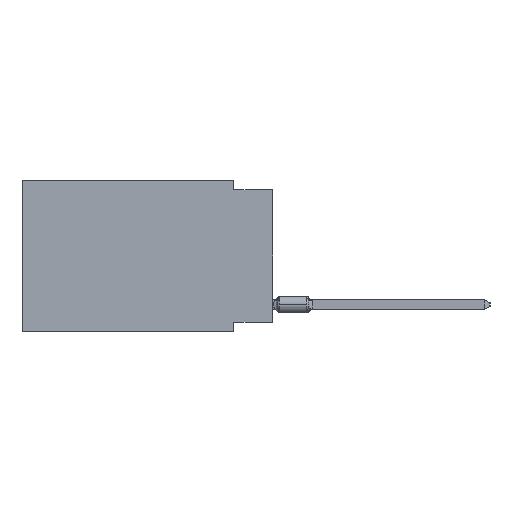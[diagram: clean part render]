
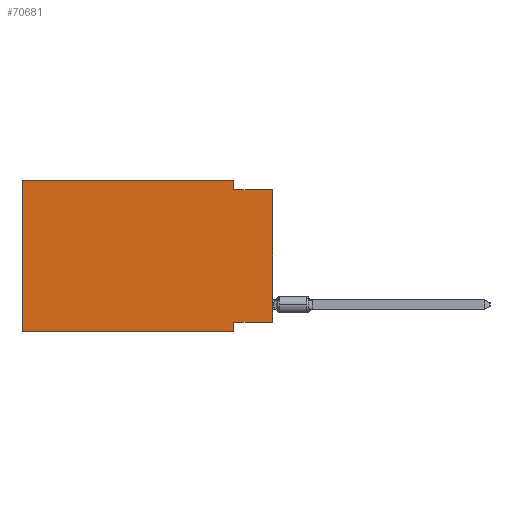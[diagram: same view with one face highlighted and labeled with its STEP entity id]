
A CAD part, left-side view. The second image highlights one B-rep face of the part: STEP entity #70681.
In plain terms, the highlighted planar face has unit normal (-1, 0, 0).
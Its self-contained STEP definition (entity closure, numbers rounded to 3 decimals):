
#711 = CARTESIAN_POINT ( 'NONE',  ( 0., 2.54, -9.271 ) ) ;
#1334 = EDGE_CURVE ( 'NONE', #35140, #52987, #44220, .T. ) ;
#3567 = DIRECTION ( 'NONE',  ( 0., 0., -1. ) ) ;
#4931 = EDGE_LOOP ( 'NONE', ( #9673, #30640, #6476, #70663, #27622, #51628, #73739, #23999 ) ) ;
#5849 = LINE ( 'NONE', #25877, #13573 ) ;
#6476 = ORIENTED_EDGE ( 'NONE', *, *, #52883, .F. ) ;
#9673 = ORIENTED_EDGE ( 'NONE', *, *, #60071, .T. ) ;
#12532 = DIRECTION ( 'NONE',  ( 0., 1., 0. ) ) ;
#13573 = VECTOR ( 'NONE', #75212, 1000. ) ;
#14777 = CARTESIAN_POINT ( 'NONE',  ( 0., 2.54, -0.635 ) ) ;
#17616 = VECTOR ( 'NONE', #43305, 1000. ) ;
#19100 = EDGE_CURVE ( 'NONE', #39209, #23145, #43921, .T. ) ;
#23145 = VERTEX_POINT ( 'NONE', #57211 ) ;
#23999 = ORIENTED_EDGE ( 'NONE', *, *, #1334, .F. ) ;
#24632 = VECTOR ( 'NONE', #60624, 1000. ) ;
#25877 = CARTESIAN_POINT ( 'NONE',  ( 0., 0., -0.635 ) ) ;
#25883 = VECTOR ( 'NONE', #12532, 1000. ) ;
#27622 = ORIENTED_EDGE ( 'NONE', *, *, #59616, .F. ) ;
#30640 = ORIENTED_EDGE ( 'NONE', *, *, #69621, .F. ) ;
#31223 = CARTESIAN_POINT ( 'NONE',  ( 0., 0., -0.635 ) ) ;
#34296 = AXIS2_PLACEMENT_3D ( 'NONE', #75398, #54502, #3567 ) ;
#34694 = LINE ( 'NONE', #53927, #24632 ) ;
#35140 = VERTEX_POINT ( 'NONE', #46275 ) ;
#35243 = CARTESIAN_POINT ( 'NONE',  ( 0., 0., 0. ) ) ;
#35932 = VERTEX_POINT ( 'NONE', #77538 ) ;
#37147 = VECTOR ( 'NONE', #43257, 1000. ) ;
#37386 = LINE ( 'NONE', #56631, #37147 ) ;
#37662 = DIRECTION ( 'NONE',  ( 0., -1., 0. ) ) ;
#39209 = VERTEX_POINT ( 'NONE', #58638 ) ;
#39528 = EDGE_CURVE ( 'NONE', #52987, #49140, #37386, .T. ) ;
#39549 = DIRECTION ( 'NONE',  ( 0., 0., 1. ) ) ;
#43257 = DIRECTION ( 'NONE',  ( 0., 0., -1. ) ) ;
#43305 = DIRECTION ( 'NONE',  ( 0., 0., -1. ) ) ;
#43921 = LINE ( 'NONE', #63602, #64338 ) ;
#44067 = CARTESIAN_POINT ( 'NONE',  ( 0., 2.54, -9.906 ) ) ;
#44220 = LINE ( 'NONE', #49255, #25883 ) ;
#45389 = LINE ( 'NONE', #70931, #74264 ) ;
#46275 = CARTESIAN_POINT ( 'NONE',  ( 0., 0., -9.271 ) ) ;
#47360 = DIRECTION ( 'NONE',  ( 0., 0., 1. ) ) ;
#49140 = VERTEX_POINT ( 'NONE', #44067 ) ;
#49255 = CARTESIAN_POINT ( 'NONE',  ( 0., 0., -9.271 ) ) ;
#50812 = LINE ( 'NONE', #55445, #17616 ) ;
#51628 = ORIENTED_EDGE ( 'NONE', *, *, #57890, .T. ) ;
#52883 = EDGE_CURVE ( 'NONE', #23145, #70148, #50812, .T. ) ;
#52987 = VERTEX_POINT ( 'NONE', #711 ) ;
#53927 = CARTESIAN_POINT ( 'NONE',  ( 0., 16.383, -9.906 ) ) ;
#54502 = DIRECTION ( 'NONE',  ( 1., 0., 0. ) ) ;
#55445 = CARTESIAN_POINT ( 'NONE',  ( 0., 2.54, 0. ) ) ;
#56139 = FACE_OUTER_BOUND ( 'NONE', #4931, .T. ) ;
#56631 = CARTESIAN_POINT ( 'NONE',  ( 0., 2.54, -9.906 ) ) ;
#57211 = CARTESIAN_POINT ( 'NONE',  ( 0., 2.54, 0. ) ) ;
#57890 = EDGE_CURVE ( 'NONE', #35932, #49140, #34694, .T. ) ;
#58638 = CARTESIAN_POINT ( 'NONE',  ( 0., 16.383, 0. ) ) ;
#59616 = EDGE_CURVE ( 'NONE', #35932, #39209, #45389, .T. ) ;
#60071 = EDGE_CURVE ( 'NONE', #35140, #73575, #78742, .T. ) ;
#60624 = DIRECTION ( 'NONE',  ( 0., -1., 0. ) ) ;
#63602 = CARTESIAN_POINT ( 'NONE',  ( 0., 16.383, 0. ) ) ;
#64338 = VECTOR ( 'NONE', #37662, 1000. ) ;
#69621 = EDGE_CURVE ( 'NONE', #70148, #73575, #5849, .T. ) ;
#70148 = VERTEX_POINT ( 'NONE', #14777 ) ;
#70663 = ORIENTED_EDGE ( 'NONE', *, *, #19100, .F. ) ;
#70681 = ADVANCED_FACE ( 'NONE', ( #56139 ), #81680, .F. ) ;
#70931 = CARTESIAN_POINT ( 'NONE',  ( 0., 16.383, 0. ) ) ;
#71688 = VECTOR ( 'NONE', #47360, 1000. ) ;
#73575 = VERTEX_POINT ( 'NONE', #31223 ) ;
#73739 = ORIENTED_EDGE ( 'NONE', *, *, #39528, .F. ) ;
#74264 = VECTOR ( 'NONE', #39549, 1000. ) ;
#75212 = DIRECTION ( 'NONE',  ( 0., -1., 0. ) ) ;
#75398 = CARTESIAN_POINT ( 'NONE',  ( 0., 16.383, 0. ) ) ;
#77538 = CARTESIAN_POINT ( 'NONE',  ( 0., 16.383, -9.906 ) ) ;
#78742 = LINE ( 'NONE', #35243, #71688 ) ;
#81680 = PLANE ( 'NONE',  #34296 ) ;
